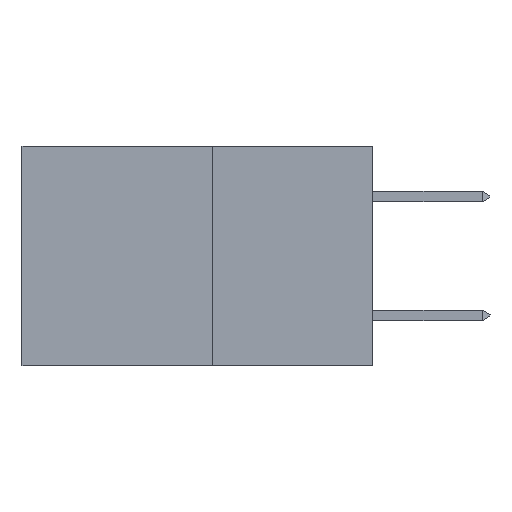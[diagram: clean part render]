
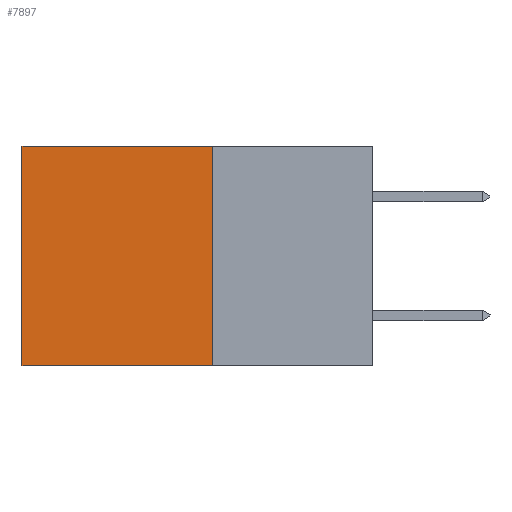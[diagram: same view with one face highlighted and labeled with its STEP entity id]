
A CAD part, left-side view. The second image highlights one B-rep face of the part: STEP entity #7897.
In plain terms, the highlighted planar face has unit normal (-1, 0, 0).
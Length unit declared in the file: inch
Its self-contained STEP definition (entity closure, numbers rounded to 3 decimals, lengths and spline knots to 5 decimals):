
#1722 = VECTOR ( 'NONE', #21593, 39.37008 ) ;
#1888 = CARTESIAN_POINT ( 'NONE',  ( 0.277, 0.59, -0.37 ) ) ;
#3713 = DIRECTION ( 'NONE',  ( 0., 0., -1. ) ) ;
#5012 = CARTESIAN_POINT ( 'NONE',  ( 0.277, 0.27, -0.37 ) ) ;
#5331 = EDGE_CURVE ( 'NONE', #24727, #31549, #26274, .T. ) ;
#6363 = AXIS2_PLACEMENT_3D ( 'NONE', #20284, #20175, #20169 ) ;
#7159 = ORIENTED_EDGE ( 'NONE', *, *, #14768, .T. ) ;
#7897 = ADVANCED_FACE ( 'NONE', ( #26460 ), #20346, .F. ) ;
#8445 = VERTEX_POINT ( 'NONE', #12727 ) ;
#8647 = CARTESIAN_POINT ( 'NONE',  ( 0.277, 0.27, -0.37 ) ) ;
#8877 = LINE ( 'NONE', #8647, #27999 ) ;
#9443 = CARTESIAN_POINT ( 'NONE',  ( 0.277, 0.59, -0.37 ) ) ;
#10132 = LINE ( 'NONE', #9443, #16816 ) ;
#11688 = EDGE_LOOP ( 'NONE', ( #31145, #14873, #31378, #7159 ) ) ;
#12185 = CARTESIAN_POINT ( 'NONE',  ( 0.277, 0.27, 0. ) ) ;
#12727 = CARTESIAN_POINT ( 'NONE',  ( 0.277, 0.59, 0. ) ) ;
#12853 = EDGE_CURVE ( 'NONE', #8445, #31549, #10132, .T. ) ;
#12918 = VERTEX_POINT ( 'NONE', #12185 ) ;
#13032 = VECTOR ( 'NONE', #15280, 39.37008 ) ;
#14768 = EDGE_CURVE ( 'NONE', #12918, #8445, #16677, .T. ) ;
#14873 = ORIENTED_EDGE ( 'NONE', *, *, #5331, .F. ) ;
#15129 = CARTESIAN_POINT ( 'NONE',  ( 0.277, 0.27, -0.37 ) ) ;
#15280 = DIRECTION ( 'NONE',  ( 0., 1., 0. ) ) ;
#16677 = LINE ( 'NONE', #18664, #1722 ) ;
#16816 = VECTOR ( 'NONE', #26902, 39.37008 ) ;
#18664 = CARTESIAN_POINT ( 'NONE',  ( 0.277, 0.27, 0. ) ) ;
#20169 = DIRECTION ( 'NONE',  ( 0., 0., -1. ) ) ;
#20175 = DIRECTION ( 'NONE',  ( 1., 0., 0. ) ) ;
#20284 = CARTESIAN_POINT ( 'NONE',  ( 0.277, 0.27, -0.37 ) ) ;
#20346 = PLANE ( 'NONE',  #6363 ) ;
#21593 = DIRECTION ( 'NONE',  ( 0., 1., 0. ) ) ;
#24727 = VERTEX_POINT ( 'NONE', #5012 ) ;
#26274 = LINE ( 'NONE', #15129, #13032 ) ;
#26460 = FACE_OUTER_BOUND ( 'NONE', #11688, .T. ) ;
#26902 = DIRECTION ( 'NONE',  ( 0., 0., -1. ) ) ;
#27999 = VECTOR ( 'NONE', #3713, 39.37008 ) ;
#31124 = EDGE_CURVE ( 'NONE', #12918, #24727, #8877, .T. ) ;
#31145 = ORIENTED_EDGE ( 'NONE', *, *, #12853, .T. ) ;
#31378 = ORIENTED_EDGE ( 'NONE', *, *, #31124, .F. ) ;
#31549 = VERTEX_POINT ( 'NONE', #1888 ) ;
